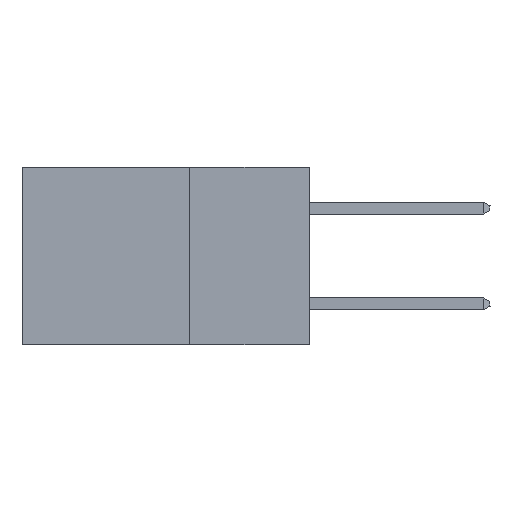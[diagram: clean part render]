
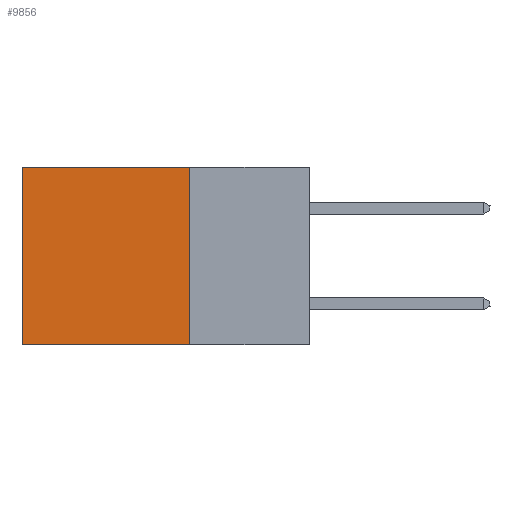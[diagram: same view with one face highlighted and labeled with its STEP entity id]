
A CAD part, left-side view. The second image highlights one B-rep face of the part: STEP entity #9856.
In plain terms, the highlighted planar face has unit normal (-1, 0, 0).
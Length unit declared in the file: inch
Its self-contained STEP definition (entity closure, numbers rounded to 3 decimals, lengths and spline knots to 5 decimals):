
#93 = ORIENTED_EDGE ( 'NONE', *, *, #2432, .T. ) ;
#2432 = EDGE_CURVE ( 'NONE', #26518, #13294, #34315, .T. ) ;
#2444 = CARTESIAN_POINT ( 'NONE',  ( 0.2875, 0.6, 0. ) ) ;
#4819 = DIRECTION ( 'NONE',  ( 0., 1., 0. ) ) ;
#6954 = EDGE_CURVE ( 'NONE', #24777, #26518, #12683, .T. ) ;
#7220 = VECTOR ( 'NONE', #4819, 39.37008 ) ;
#8941 = EDGE_CURVE ( 'NONE', #24777, #37533, #10562, .T. ) ;
#9633 = VECTOR ( 'NONE', #32447, 39.37008 ) ;
#9856 = ADVANCED_FACE ( 'NONE', ( #14162 ), #13791, .F. ) ;
#10562 = LINE ( 'NONE', #14531, #9633 ) ;
#11249 = VECTOR ( 'NONE', #17279, 39.37008 ) ;
#12683 = LINE ( 'NONE', #13407, #7220 ) ;
#12758 = CARTESIAN_POINT ( 'NONE',  ( 0.2875, 0.6, 0. ) ) ;
#13294 = VERTEX_POINT ( 'NONE', #34074 ) ;
#13407 = CARTESIAN_POINT ( 'NONE',  ( 0.2875, 0.25, 0. ) ) ;
#13791 = PLANE ( 'NONE',  #33167 ) ;
#14162 = FACE_OUTER_BOUND ( 'NONE', #26885, .T. ) ;
#14531 = CARTESIAN_POINT ( 'NONE',  ( 0.2875, 0.25, 0. ) ) ;
#17279 = DIRECTION ( 'NONE',  ( 0., 0., -1. ) ) ;
#19612 = DIRECTION ( 'NONE',  ( 0., 0., -1. ) ) ;
#21002 = ORIENTED_EDGE ( 'NONE', *, *, #8941, .F. ) ;
#22613 = CARTESIAN_POINT ( 'NONE',  ( 0.2875, 0.25, 0. ) ) ;
#24777 = VERTEX_POINT ( 'NONE', #22613 ) ;
#25817 = LINE ( 'NONE', #27694, #29518 ) ;
#26518 = VERTEX_POINT ( 'NONE', #12758 ) ;
#26885 = EDGE_LOOP ( 'NONE', ( #93, #28651, #21002, #34275 ) ) ;
#27455 = DIRECTION ( 'NONE',  ( 0., 1., 0. ) ) ;
#27694 = CARTESIAN_POINT ( 'NONE',  ( 0.2875, 0.25, -0.37 ) ) ;
#28651 = ORIENTED_EDGE ( 'NONE', *, *, #36106, .F. ) ;
#29518 = VECTOR ( 'NONE', #27455, 39.37008 ) ;
#31540 = CARTESIAN_POINT ( 'NONE',  ( 0.2875, 0.25, -0.37 ) ) ;
#32447 = DIRECTION ( 'NONE',  ( 0., 0., -1. ) ) ;
#33167 = AXIS2_PLACEMENT_3D ( 'NONE', #36905, #37406, #19612 ) ;
#34074 = CARTESIAN_POINT ( 'NONE',  ( 0.2875, 0.6, -0.37 ) ) ;
#34275 = ORIENTED_EDGE ( 'NONE', *, *, #6954, .T. ) ;
#34315 = LINE ( 'NONE', #2444, #11249 ) ;
#36106 = EDGE_CURVE ( 'NONE', #37533, #13294, #25817, .T. ) ;
#36905 = CARTESIAN_POINT ( 'NONE',  ( 0.2875, 0.25, 0. ) ) ;
#37406 = DIRECTION ( 'NONE',  ( 1., 0., 0. ) ) ;
#37533 = VERTEX_POINT ( 'NONE', #31540 ) ;
